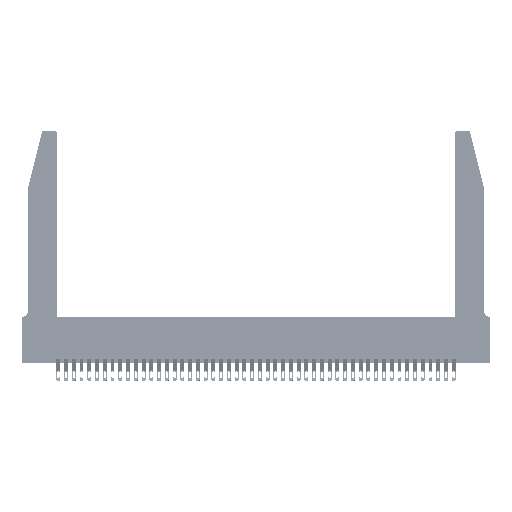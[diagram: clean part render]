
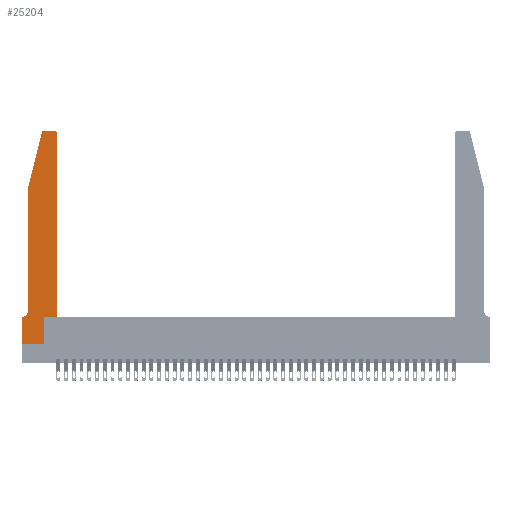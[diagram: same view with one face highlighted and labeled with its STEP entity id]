
A CAD part, top view. The second image highlights one B-rep face of the part: STEP entity #25204.
In plain terms, the highlighted planar face has unit normal (0, 0, 1).
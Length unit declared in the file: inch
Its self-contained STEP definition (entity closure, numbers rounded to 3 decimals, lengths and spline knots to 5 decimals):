
#66 = ORIENTED_EDGE ( 'NONE', *, *, #23588, .T. ) ;
#420 = LINE ( 'NONE', #24879, #17688 ) ;
#973 = DIRECTION ( 'NONE',  ( 1., 0., 0. ) ) ;
#1192 = ORIENTED_EDGE ( 'NONE', *, *, #29779, .T. ) ;
#2474 = EDGE_CURVE ( 'NONE', #14565, #39191, #33590, .T. ) ;
#2567 = LINE ( 'NONE', #5316, #33330 ) ;
#3287 = EDGE_CURVE ( 'NONE', #7662, #3338, #17850, .T. ) ;
#3338 = VERTEX_POINT ( 'NONE', #33680 ) ;
#3797 = CARTESIAN_POINT ( 'NONE',  ( 0.2865, 0., 0.37 ) ) ;
#4228 = CARTESIAN_POINT ( 'NONE',  ( 0.4205, 2.72, 0.37 ) ) ;
#5316 = CARTESIAN_POINT ( 'NONE',  ( 0., 0., 0.37 ) ) ;
#5581 = CARTESIAN_POINT ( 'NONE',  ( 0.0755, 2., 0.37 ) ) ;
#5610 = CARTESIAN_POINT ( 'NONE',  ( 0.0755, 2., 0.37 ) ) ;
#5921 = ORIENTED_EDGE ( 'NONE', *, *, #30231, .T. ) ;
#6028 = DIRECTION ( 'NONE',  ( 0., -1., 0. ) ) ;
#6258 = CARTESIAN_POINT ( 'NONE',  ( 0.2865, 0.35, 0.37 ) ) ;
#6289 = CARTESIAN_POINT ( 'NONE',  ( 0., 0.35, 0.37 ) ) ;
#6948 = ORIENTED_EDGE ( 'NONE', *, *, #27506, .T. ) ;
#7662 = VERTEX_POINT ( 'NONE', #17839 ) ;
#7898 = DIRECTION ( 'NONE',  ( -1., 0., 0. ) ) ;
#8415 = DIRECTION ( 'NONE',  ( 1., 0., 0. ) ) ;
#8572 = PLANE ( 'NONE',  #42296 ) ;
#8616 = VERTEX_POINT ( 'NONE', #12776 ) ;
#8727 = CARTESIAN_POINT ( 'NONE',  ( 0., 0.35, 0.37 ) ) ;
#8801 = DIRECTION ( 'NONE',  ( 1., 0., 0. ) ) ;
#9256 = VERTEX_POINT ( 'NONE', #22781 ) ;
#9401 = EDGE_CURVE ( 'NONE', #32595, #10811, #37424, .T. ) ;
#9435 = VERTEX_POINT ( 'NONE', #6258 ) ;
#10811 = VERTEX_POINT ( 'NONE', #22144 ) ;
#11045 = CARTESIAN_POINT ( 'NONE',  ( 0.0755, 0.35, 0.37 ) ) ;
#11878 = AXIS2_PLACEMENT_3D ( 'NONE', #13327, #20331, #30731 ) ;
#12178 = DIRECTION ( 'NONE',  ( 0., 0., 1. ) ) ;
#12635 = CARTESIAN_POINT ( 'NONE',  ( 0.4505, 0.35, 0.37 ) ) ;
#12776 = CARTESIAN_POINT ( 'NONE',  ( 0.0755, 2., 0.37 ) ) ;
#13327 = CARTESIAN_POINT ( 'NONE',  ( 0.284, 2.72, 0.37 ) ) ;
#13893 = EDGE_CURVE ( 'NONE', #41512, #21941, #23165, .T. ) ;
#14434 = LINE ( 'NONE', #24685, #31741 ) ;
#14565 = VERTEX_POINT ( 'NONE', #34100 ) ;
#15481 = DIRECTION ( 'NONE',  ( 0., -1., 0. ) ) ;
#15679 = LINE ( 'NONE', #38788, #32937 ) ;
#17688 = VECTOR ( 'NONE', #41939, 39.37008 ) ;
#17839 = CARTESIAN_POINT ( 'NONE',  ( 0.0755, 0.42, 0.37 ) ) ;
#17850 = CIRCLE ( 'NONE', #25335, 0.07 ) ;
#18900 = ORIENTED_EDGE ( 'NONE', *, *, #29582, .T. ) ;
#19030 = ORIENTED_EDGE ( 'NONE', *, *, #2474, .T. ) ;
#20331 = DIRECTION ( 'NONE',  ( 0., 0., 1. ) ) ;
#21067 = VECTOR ( 'NONE', #6028, 39.37008 ) ;
#21469 = DIRECTION ( 'NONE',  ( 1., 0., 0. ) ) ;
#21941 = VERTEX_POINT ( 'NONE', #25084 ) ;
#22144 = CARTESIAN_POINT ( 'NONE',  ( 0.25487, 2.72718, 0.37 ) ) ;
#22710 = LINE ( 'NONE', #12635, #32945 ) ;
#22781 = CARTESIAN_POINT ( 'NONE',  ( 0.4505, 0.35, 0.37 ) ) ;
#22900 = CARTESIAN_POINT ( 'NONE',  ( 0.4505, 2.72, 0.37 ) ) ;
#23165 = CIRCLE ( 'NONE', #27913, 0.03 ) ;
#23518 = VERTEX_POINT ( 'NONE', #6289 ) ;
#23588 = EDGE_CURVE ( 'NONE', #9435, #9256, #15679, .T. ) ;
#23928 = ORIENTED_EDGE ( 'NONE', *, *, #37728, .T. ) ;
#24641 = EDGE_CURVE ( 'NONE', #23518, #14565, #2567, .T. ) ;
#24685 = CARTESIAN_POINT ( 'NONE',  ( 0.2605, 2.75, 0.37 ) ) ;
#24879 = CARTESIAN_POINT ( 'NONE',  ( 0.2865, 0.35, 0.37 ) ) ;
#24997 = DIRECTION ( 'NONE',  ( -1., 0., 0. ) ) ;
#25084 = CARTESIAN_POINT ( 'NONE',  ( 0.4205, 2.75, 0.37 ) ) ;
#25204 = ADVANCED_FACE ( 'NONE', ( #38586 ), #8572, .T. ) ;
#25335 = AXIS2_PLACEMENT_3D ( 'NONE', #35395, #26105, #43877 ) ;
#26105 = DIRECTION ( 'NONE',  ( 0., 0., -1. ) ) ;
#26842 = ORIENTED_EDGE ( 'NONE', *, *, #35624, .T. ) ;
#27172 = LINE ( 'NONE', #11045, #31472 ) ;
#27210 = CARTESIAN_POINT ( 'NONE',  ( 0.284, 2.75, 0.37 ) ) ;
#27506 = EDGE_CURVE ( 'NONE', #3338, #23518, #27172, .T. ) ;
#27913 = AXIS2_PLACEMENT_3D ( 'NONE', #4228, #28575, #21469 ) ;
#28575 = DIRECTION ( 'NONE',  ( 0., 0., 1. ) ) ;
#29443 = ORIENTED_EDGE ( 'NONE', *, *, #9401, .T. ) ;
#29556 = CARTESIAN_POINT ( 'NONE',  ( 0., 0., 0.37 ) ) ;
#29582 = EDGE_CURVE ( 'NONE', #8616, #7662, #43643, .T. ) ;
#29779 = EDGE_CURVE ( 'NONE', #39191, #9435, #420, .T. ) ;
#30231 = EDGE_CURVE ( 'NONE', #21941, #32595, #14434, .T. ) ;
#30731 = DIRECTION ( 'NONE',  ( 1., 0., 0. ) ) ;
#31472 = VECTOR ( 'NONE', #7898, 39.37008 ) ;
#31694 = ORIENTED_EDGE ( 'NONE', *, *, #24641, .T. ) ;
#31741 = VECTOR ( 'NONE', #24997, 39.37008 ) ;
#32595 = VERTEX_POINT ( 'NONE', #27210 ) ;
#32937 = VECTOR ( 'NONE', #973, 39.37008 ) ;
#32945 = VECTOR ( 'NONE', #40218, 39.37008 ) ;
#33330 = VECTOR ( 'NONE', #15481, 39.37008 ) ;
#33590 = LINE ( 'NONE', #29556, #38347 ) ;
#33680 = CARTESIAN_POINT ( 'NONE',  ( 0.0055, 0.35, 0.37 ) ) ;
#34100 = CARTESIAN_POINT ( 'NONE',  ( 0., 0., 0.37 ) ) ;
#35395 = CARTESIAN_POINT ( 'NONE',  ( 0.0055, 0.42, 0.37 ) ) ;
#35595 = LINE ( 'NONE', #5610, #36680 ) ;
#35624 = EDGE_CURVE ( 'NONE', #9256, #41512, #22710, .T. ) ;
#36680 = VECTOR ( 'NONE', #36796, 39.37008 ) ;
#36796 = DIRECTION ( 'NONE',  ( -0.239, -0.971, 0. ) ) ;
#37424 = CIRCLE ( 'NONE', #11878, 0.03 ) ;
#37728 = EDGE_CURVE ( 'NONE', #10811, #8616, #35595, .T. ) ;
#38347 = VECTOR ( 'NONE', #8801, 39.37008 ) ;
#38586 = FACE_OUTER_BOUND ( 'NONE', #44565, .T. ) ;
#38788 = CARTESIAN_POINT ( 'NONE',  ( 0.4505, 0.35, 0.37 ) ) ;
#39171 = ORIENTED_EDGE ( 'NONE', *, *, #3287, .T. ) ;
#39191 = VERTEX_POINT ( 'NONE', #3797 ) ;
#40218 = DIRECTION ( 'NONE',  ( 0., 1., 0. ) ) ;
#41512 = VERTEX_POINT ( 'NONE', #22900 ) ;
#41939 = DIRECTION ( 'NONE',  ( 0., 1., 0. ) ) ;
#42296 = AXIS2_PLACEMENT_3D ( 'NONE', #8727, #12178, #8415 ) ;
#42691 = ORIENTED_EDGE ( 'NONE', *, *, #13893, .T. ) ;
#43643 = LINE ( 'NONE', #5581, #21067 ) ;
#43877 = DIRECTION ( 'NONE',  ( -1., 0., 0. ) ) ;
#44565 = EDGE_LOOP ( 'NONE', ( #5921, #29443, #23928, #18900, #39171, #6948, #31694, #19030, #1192, #66, #26842, #42691 ) ) ;
